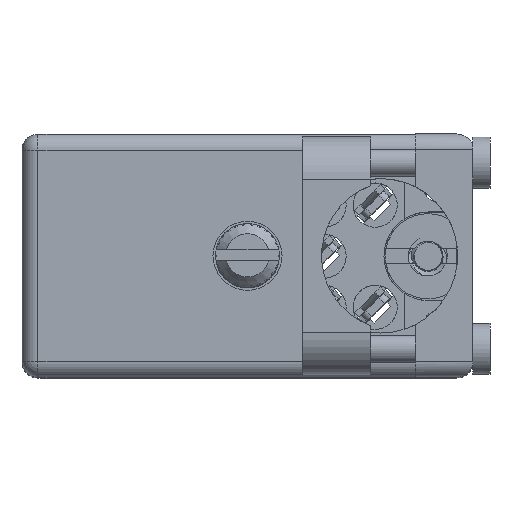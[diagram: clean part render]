
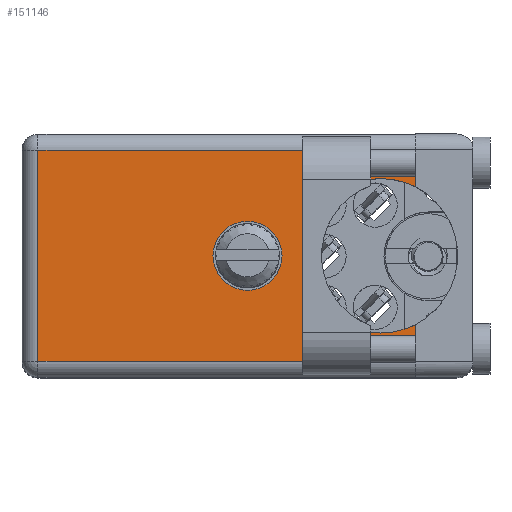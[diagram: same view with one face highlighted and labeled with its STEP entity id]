
A CAD part, top view. The second image highlights one B-rep face of the part: STEP entity #151146.
In plain terms, the highlighted face is planar.
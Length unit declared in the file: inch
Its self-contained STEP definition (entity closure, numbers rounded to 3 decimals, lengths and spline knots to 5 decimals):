
#239 = VERTEX_POINT ( 'NONE', #43272 ) ;
#1322 = VERTEX_POINT ( 'NONE', #175229 ) ;
#4098 = AXIS2_PLACEMENT_3D ( 'NONE', #7541, #186213, #34158 ) ;
#4432 = VERTEX_POINT ( 'NONE', #147271 ) ;
#6202 = EDGE_CURVE ( 'NONE', #175537, #60172, #19352, .T. ) ;
#6931 = CARTESIAN_POINT ( 'NONE',  ( 1.155, 0.906, -0.047 ) ) ;
#7114 = DIRECTION ( 'NONE',  ( 0., 0., 1. ) ) ;
#7541 = CARTESIAN_POINT ( 'NONE',  ( 1.053, 0.906, -0.3575 ) ) ;
#8362 = EDGE_LOOP ( 'NONE', ( #193861, #51805, #143783, #101879, #19064, #117795, #75179, #163343 ) ) ;
#8892 = LINE ( 'NONE', #6931, #81076 ) ;
#10389 = CARTESIAN_POINT ( 'NONE',  ( 1.155, 0.906, 0. ) ) ;
#15362 = CARTESIAN_POINT ( 'NONE',  ( 0., 0.906, -0.715 ) ) ;
#18692 = DIRECTION ( 'NONE',  ( -1., 0., 0. ) ) ;
#19064 = ORIENTED_EDGE ( 'NONE', *, *, #177324, .F. ) ;
#19352 = CIRCLE ( 'NONE', #44564, 0.227 ) ;
#24998 = VERTEX_POINT ( 'NONE', #105179 ) ;
#29061 = CARTESIAN_POINT ( 'NONE',  ( 0.6625, 0.906, -0.256 ) ) ;
#31205 = CARTESIAN_POINT ( 'NONE',  ( 0.047, 0.906, -0.715 ) ) ;
#34158 = DIRECTION ( 'NONE',  ( 0., 0., 1. ) ) ;
#36902 = EDGE_CURVE ( 'NONE', #4432, #1322, #89305, .T. ) ;
#36974 = CIRCLE ( 'NONE', #147430, 0.1015 ) ;
#42979 = PLANE ( 'NONE',  #97365 ) ;
#43272 = CARTESIAN_POINT ( 'NONE',  ( 1.155, 0.906, -0.047 ) ) ;
#44564 = AXIS2_PLACEMENT_3D ( 'NONE', #114452, #100605, #173702 ) ;
#45137 = CARTESIAN_POINT ( 'NONE',  ( 1.155, 0.906, 0. ) ) ;
#51805 = ORIENTED_EDGE ( 'NONE', *, *, #130278, .T. ) ;
#52480 = DIRECTION ( 'NONE',  ( 0., 1., 0. ) ) ;
#56585 = DIRECTION ( 'NONE',  ( 0., 0., 1. ) ) ;
#60172 = VERTEX_POINT ( 'NONE', #160707 ) ;
#61724 = FACE_OUTER_BOUND ( 'NONE', #8362, .T. ) ;
#62352 = EDGE_CURVE ( 'NONE', #108219, #239, #8892, .T. ) ;
#62911 = DIRECTION ( 'NONE',  ( 0., 0., 1. ) ) ;
#64109 = LINE ( 'NONE', #151103, #136080 ) ;
#74834 = LINE ( 'NONE', #45137, #90606 ) ;
#75179 = ORIENTED_EDGE ( 'NONE', *, *, #134144, .F. ) ;
#81076 = VECTOR ( 'NONE', #188546, 39.37008 ) ;
#81511 = EDGE_CURVE ( 'NONE', #131718, #4432, #74834, .T. ) ;
#82225 = CARTESIAN_POINT ( 'NONE',  ( 1.053, 0.906, -0.1305 ) ) ;
#89305 = CIRCLE ( 'NONE', #4098, 0.227 ) ;
#90606 = VECTOR ( 'NONE', #62911, 39.37008 ) ;
#92206 = AXIS2_PLACEMENT_3D ( 'NONE', #157192, #52480, #7114 ) ;
#94367 = VERTEX_POINT ( 'NONE', #29061 ) ;
#97365 = AXIS2_PLACEMENT_3D ( 'NONE', #15362, #119040, #193112 ) ;
#99663 = CIRCLE ( 'NONE', #187997, 0.1015 ) ;
#100605 = DIRECTION ( 'NONE',  ( 0., 1., 0. ) ) ;
#101035 = DIRECTION ( 'NONE',  ( 0., 1., 0. ) ) ;
#101879 = ORIENTED_EDGE ( 'NONE', *, *, #62352, .T. ) ;
#102368 = VECTOR ( 'NONE', #176230, 39.37008 ) ;
#105179 = CARTESIAN_POINT ( 'NONE',  ( 0.047, 0.906, -0.668 ) ) ;
#106743 = EDGE_CURVE ( 'NONE', #24998, #108219, #134962, .T. ) ;
#108219 = VERTEX_POINT ( 'NONE', #186838 ) ;
#114452 = CARTESIAN_POINT ( 'NONE',  ( 1.053, 0.906, -0.3575 ) ) ;
#115041 = LINE ( 'NONE', #10389, #102368 ) ;
#115844 = CARTESIAN_POINT ( 'NONE',  ( 0.6625, 0.906, -0.3575 ) ) ;
#117795 = ORIENTED_EDGE ( 'NONE', *, *, #6202, .F. ) ;
#119040 = DIRECTION ( 'NONE',  ( 0., 1., 0. ) ) ;
#119059 = DIRECTION ( 'NONE',  ( 0., 0., 1. ) ) ;
#130278 = EDGE_CURVE ( 'NONE', #131718, #24998, #64109, .T. ) ;
#131718 = VERTEX_POINT ( 'NONE', #157193 ) ;
#134144 = EDGE_CURVE ( 'NONE', #1322, #175537, #174085, .T. ) ;
#134962 = LINE ( 'NONE', #31205, #164156 ) ;
#136080 = VECTOR ( 'NONE', #18692, 39.37008 ) ;
#136827 = DIRECTION ( 'NONE',  ( 0., 1., 0. ) ) ;
#139292 = EDGE_LOOP ( 'NONE', ( #166230, #142346 ) ) ;
#142346 = ORIENTED_EDGE ( 'NONE', *, *, #186621, .F. ) ;
#143783 = ORIENTED_EDGE ( 'NONE', *, *, #106743, .T. ) ;
#147271 = CARTESIAN_POINT ( 'NONE',  ( 1.155, 0.906, -0.56029 ) ) ;
#147405 = EDGE_CURVE ( 'NONE', #94367, #171413, #36974, .T. ) ;
#147430 = AXIS2_PLACEMENT_3D ( 'NONE', #164516, #136827, #119059 ) ;
#150661 = FACE_BOUND ( 'NONE', #139292, .T. ) ;
#151103 = CARTESIAN_POINT ( 'NONE',  ( 0., 0.906, -0.668 ) ) ;
#151146 = ADVANCED_FACE ( 'NONE', ( #61724, #150661 ), #42979, .T. ) ;
#157192 = CARTESIAN_POINT ( 'NONE',  ( 1.053, 0.906, -0.3575 ) ) ;
#157193 = CARTESIAN_POINT ( 'NONE',  ( 1.155, 0.906, -0.668 ) ) ;
#160707 = CARTESIAN_POINT ( 'NONE',  ( 1.155, 0.906, -0.15471 ) ) ;
#163343 = ORIENTED_EDGE ( 'NONE', *, *, #36902, .F. ) ;
#164156 = VECTOR ( 'NONE', #180319, 39.37008 ) ;
#164516 = CARTESIAN_POINT ( 'NONE',  ( 0.6625, 0.906, -0.3575 ) ) ;
#166230 = ORIENTED_EDGE ( 'NONE', *, *, #147405, .F. ) ;
#171413 = VERTEX_POINT ( 'NONE', #177685 ) ;
#173702 = DIRECTION ( 'NONE',  ( 0., 0., 1. ) ) ;
#174085 = CIRCLE ( 'NONE', #92206, 0.227 ) ;
#175229 = CARTESIAN_POINT ( 'NONE',  ( 1.053, 0.906, -0.5845 ) ) ;
#175537 = VERTEX_POINT ( 'NONE', #82225 ) ;
#176230 = DIRECTION ( 'NONE',  ( 0., 0., 1. ) ) ;
#177324 = EDGE_CURVE ( 'NONE', #60172, #239, #115041, .T. ) ;
#177685 = CARTESIAN_POINT ( 'NONE',  ( 0.6625, 0.906, -0.459 ) ) ;
#180319 = DIRECTION ( 'NONE',  ( 0., 0., 1. ) ) ;
#186213 = DIRECTION ( 'NONE',  ( 0., 1., 0. ) ) ;
#186621 = EDGE_CURVE ( 'NONE', #171413, #94367, #99663, .T. ) ;
#186838 = CARTESIAN_POINT ( 'NONE',  ( 0.047, 0.906, -0.047 ) ) ;
#187997 = AXIS2_PLACEMENT_3D ( 'NONE', #115844, #101035, #56585 ) ;
#188546 = DIRECTION ( 'NONE',  ( 1., 0., 0. ) ) ;
#193112 = DIRECTION ( 'NONE',  ( 0., 0., 1. ) ) ;
#193861 = ORIENTED_EDGE ( 'NONE', *, *, #81511, .F. ) ;
